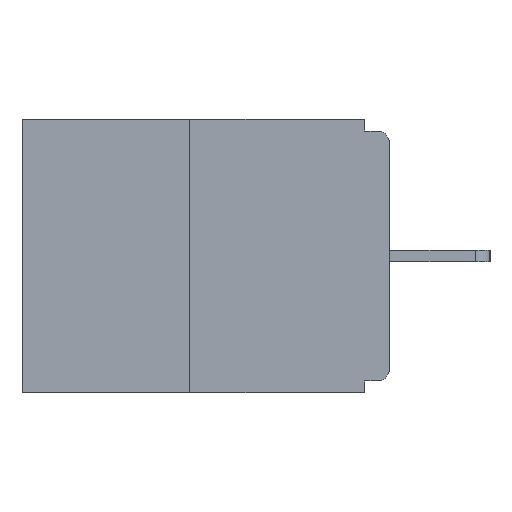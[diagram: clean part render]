
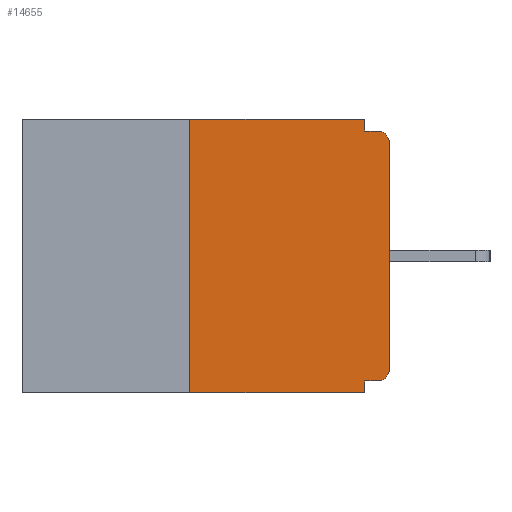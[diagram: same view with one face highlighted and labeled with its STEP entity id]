
A CAD part, left-side view. The second image highlights one B-rep face of the part: STEP entity #14655.
In plain terms, the highlighted planar face has unit normal (-1, 0, 0).
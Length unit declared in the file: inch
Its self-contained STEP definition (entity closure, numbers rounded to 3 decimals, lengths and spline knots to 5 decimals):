
#24 = DIRECTION ( 'NONE',  ( 0., -1., 0. ) ) ;
#402 = CARTESIAN_POINT ( 'NONE',  ( 0., 0.031, 0. ) ) ;
#432 = LINE ( 'NONE', #18304, #15307 ) ;
#972 = VERTEX_POINT ( 'NONE', #7543 ) ;
#1195 = LINE ( 'NONE', #402, #16020 ) ;
#1411 = EDGE_CURVE ( 'NONE', #14745, #4783, #11292, .T. ) ;
#1823 = EDGE_CURVE ( 'NONE', #15801, #7857, #15907, .T. ) ;
#1905 = EDGE_CURVE ( 'NONE', #4174, #2219, #4983, .T. ) ;
#1920 = DIRECTION ( 'NONE',  ( 0., 0., -1. ) ) ;
#2134 = FACE_OUTER_BOUND ( 'NONE', #3347, .T. ) ;
#2219 = VERTEX_POINT ( 'NONE', #12823 ) ;
#2260 = DIRECTION ( 'NONE',  ( 0., 1., 0. ) ) ;
#2606 = CARTESIAN_POINT ( 'NONE',  ( 0., 0., -0.313 ) ) ;
#2867 = DIRECTION ( 'NONE',  ( -1., 0., 0. ) ) ;
#3174 = AXIS2_PLACEMENT_3D ( 'NONE', #12487, #3865, #13918 ) ;
#3347 = EDGE_LOOP ( 'NONE', ( #4934, #12561, #16309, #5810, #6257, #17630, #10527, #7139, #14763, #15206 ) ) ;
#3350 = CARTESIAN_POINT ( 'NONE',  ( 0., 0.46, 0. ) ) ;
#3453 = VECTOR ( 'NONE', #5661, 39.37008 ) ;
#3786 = AXIS2_PLACEMENT_3D ( 'NONE', #11415, #2867, #12826 ) ;
#3865 = DIRECTION ( 'NONE',  ( -1., 0., 0. ) ) ;
#4174 = VERTEX_POINT ( 'NONE', #8764 ) ;
#4420 = CARTESIAN_POINT ( 'NONE',  ( 0., 0.46, 0. ) ) ;
#4692 = LINE ( 'NONE', #4420, #8471 ) ;
#4701 = CARTESIAN_POINT ( 'NONE',  ( 0., 0.25, -0.343 ) ) ;
#4783 = VERTEX_POINT ( 'NONE', #7569 ) ;
#4830 = EDGE_CURVE ( 'NONE', #8593, #18560, #1195, .T. ) ;
#4934 = ORIENTED_EDGE ( 'NONE', *, *, #18439, .F. ) ;
#4983 = CIRCLE ( 'NONE', #3786, 0.015 ) ;
#5661 = DIRECTION ( 'NONE',  ( 0., -1., 0. ) ) ;
#5780 = EDGE_CURVE ( 'NONE', #4783, #972, #432, .T. ) ;
#5810 = ORIENTED_EDGE ( 'NONE', *, *, #5780, .F. ) ;
#5842 = LINE ( 'NONE', #15556, #13043 ) ;
#6236 = DIRECTION ( 'NONE',  ( 1., 0., 0. ) ) ;
#6257 = ORIENTED_EDGE ( 'NONE', *, *, #1411, .F. ) ;
#6812 = CARTESIAN_POINT ( 'NONE',  ( 0., 0.25, 0. ) ) ;
#6901 = DIRECTION ( 'NONE',  ( 0., -1., 0. ) ) ;
#7139 = ORIENTED_EDGE ( 'NONE', *, *, #1905, .T. ) ;
#7417 = VECTOR ( 'NONE', #2260, 39.37008 ) ;
#7527 = CARTESIAN_POINT ( 'NONE',  ( 0., 0.031, -0.015 ) ) ;
#7535 = AXIS2_PLACEMENT_3D ( 'NONE', #3350, #6236, #16226 ) ;
#7543 = CARTESIAN_POINT ( 'NONE',  ( 0., 0.031, -0.343 ) ) ;
#7569 = CARTESIAN_POINT ( 'NONE',  ( 0., 0.031, -0.328 ) ) ;
#7857 = VERTEX_POINT ( 'NONE', #6812 ) ;
#8295 = VECTOR ( 'NONE', #9217, 39.37008 ) ;
#8471 = VECTOR ( 'NONE', #24, 39.37008 ) ;
#8593 = VERTEX_POINT ( 'NONE', #18544 ) ;
#8764 = CARTESIAN_POINT ( 'NONE',  ( 0., 0., -0.03 ) ) ;
#9217 = DIRECTION ( 'NONE',  ( 0., 0., 1. ) ) ;
#9290 = CARTESIAN_POINT ( 'NONE',  ( 0., 0.25, 0. ) ) ;
#9984 = CARTESIAN_POINT ( 'NONE',  ( 0., 0., -0.015 ) ) ;
#10527 = ORIENTED_EDGE ( 'NONE', *, *, #11253, .T. ) ;
#10592 = EDGE_CURVE ( 'NONE', #15801, #972, #17023, .T. ) ;
#11253 = EDGE_CURVE ( 'NONE', #17036, #4174, #5842, .T. ) ;
#11292 = LINE ( 'NONE', #12422, #7417 ) ;
#11294 = DIRECTION ( 'NONE',  ( 0., 0., -1. ) ) ;
#11415 = CARTESIAN_POINT ( 'NONE',  ( 0., 0.015, -0.03 ) ) ;
#12422 = CARTESIAN_POINT ( 'NONE',  ( 0., 0., -0.328 ) ) ;
#12487 = CARTESIAN_POINT ( 'NONE',  ( 0., 0.015, -0.313 ) ) ;
#12561 = ORIENTED_EDGE ( 'NONE', *, *, #1823, .F. ) ;
#12567 = CIRCLE ( 'NONE', #3174, 0.015 ) ;
#12823 = CARTESIAN_POINT ( 'NONE',  ( 0., 0.015, -0.015 ) ) ;
#12826 = DIRECTION ( 'NONE',  ( 0., 0., -1. ) ) ;
#13043 = VECTOR ( 'NONE', #16991, 39.37008 ) ;
#13918 = DIRECTION ( 'NONE',  ( 0., 0., -1. ) ) ;
#14655 = ADVANCED_FACE ( 'NONE', ( #2134 ), #14800, .F. ) ;
#14745 = VERTEX_POINT ( 'NONE', #16344 ) ;
#14763 = ORIENTED_EDGE ( 'NONE', *, *, #15010, .F. ) ;
#14800 = PLANE ( 'NONE',  #7535 ) ;
#15010 = EDGE_CURVE ( 'NONE', #18560, #2219, #18628, .T. ) ;
#15206 = ORIENTED_EDGE ( 'NONE', *, *, #4830, .F. ) ;
#15307 = VECTOR ( 'NONE', #11294, 39.37008 ) ;
#15465 = CARTESIAN_POINT ( 'NONE',  ( 0., 0.46, -0.343 ) ) ;
#15556 = CARTESIAN_POINT ( 'NONE',  ( 0., 0., 0. ) ) ;
#15801 = VERTEX_POINT ( 'NONE', #4701 ) ;
#15907 = LINE ( 'NONE', #9290, #8295 ) ;
#16020 = VECTOR ( 'NONE', #1920, 39.37008 ) ;
#16226 = DIRECTION ( 'NONE',  ( 0., 0., -1. ) ) ;
#16309 = ORIENTED_EDGE ( 'NONE', *, *, #10592, .T. ) ;
#16344 = CARTESIAN_POINT ( 'NONE',  ( 0., 0.015, -0.328 ) ) ;
#16588 = VECTOR ( 'NONE', #6901, 39.37008 ) ;
#16991 = DIRECTION ( 'NONE',  ( 0., 0., 1. ) ) ;
#17023 = LINE ( 'NONE', #15465, #16588 ) ;
#17036 = VERTEX_POINT ( 'NONE', #2606 ) ;
#17630 = ORIENTED_EDGE ( 'NONE', *, *, #18179, .T. ) ;
#18179 = EDGE_CURVE ( 'NONE', #14745, #17036, #12567, .T. ) ;
#18304 = CARTESIAN_POINT ( 'NONE',  ( 0., 0.031, -0.343 ) ) ;
#18439 = EDGE_CURVE ( 'NONE', #7857, #8593, #4692, .T. ) ;
#18544 = CARTESIAN_POINT ( 'NONE',  ( 0., 0.031, 0. ) ) ;
#18560 = VERTEX_POINT ( 'NONE', #7527 ) ;
#18628 = LINE ( 'NONE', #9984, #3453 ) ;
